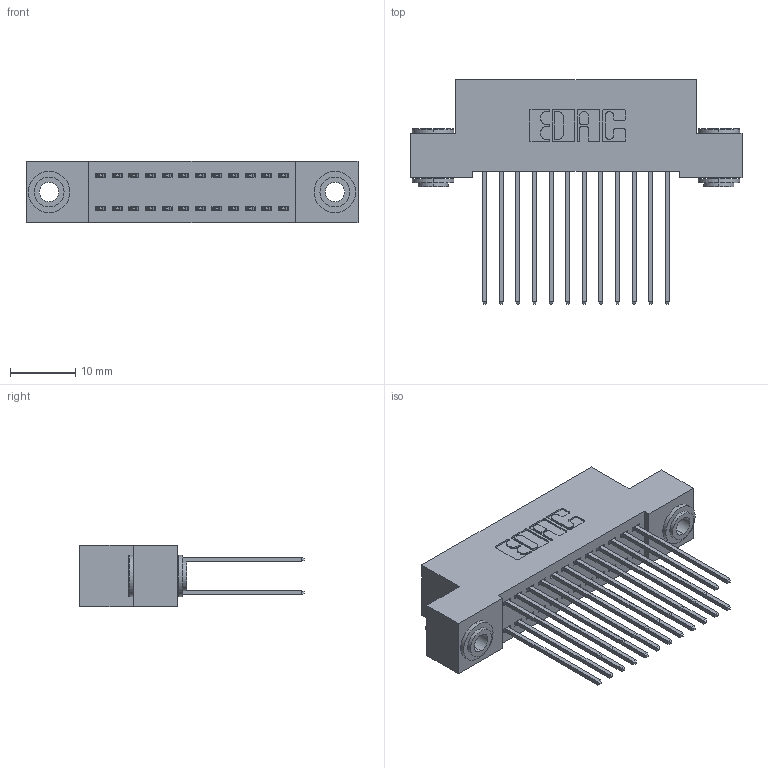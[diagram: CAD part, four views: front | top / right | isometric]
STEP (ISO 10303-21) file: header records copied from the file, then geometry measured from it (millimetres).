
FILE_DESCRIPTION (( 'STEP AP203' ), '1' );
FILE_NAME ('342-024-541-203.STEP', '2019-10-01T23:55:22', ( '' ), ( '' ), 'SwSTEP 2.0', 'SolidWorks 2016', '' );
FILE_SCHEMA (( 'CONFIG_CONTROL_DESIGN' ));
Length unit declared in the file: inch
Products named in the file (4): 345-292-001_345-293-141; 342-250-002_345-250-002-102; 342-024-541-203; 342 Part_.156 TH
Assembly tree (27 placements, depth 2):
  342-024-541-203
    342 Part_.156 TH
    345-292-001_345-293-141  x24
    342-250-002_345-250-002-102  x2
Bounding box: 50.8 x 34.3 x 9.4 mm (x, y, z)
Volume: 4582.9 mm3; surface area: 7557.3 mm2
Topology: 27 solids, 27 shells, 1396 faces, 4095 edges, 2694 vertices
Faces by surface type: plane 940, cylinder 448, cone 8
Entity records: 12136 total; most frequent: CARTESIAN_POINT 2021, ORIENTED_EDGE 1950, DIRECTION 1813, EDGE_CURVE 975, LINE 823, VECTOR 823, VERTEX_POINT 646, AXIS2_PLACEMENT_3D 495
